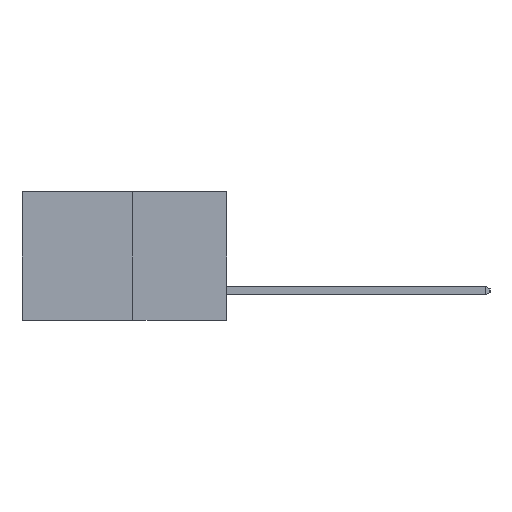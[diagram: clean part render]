
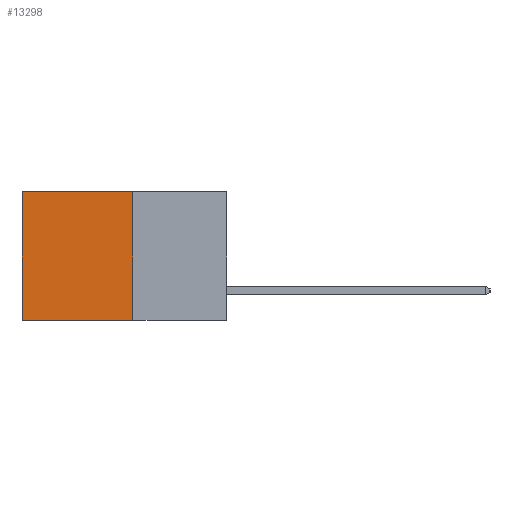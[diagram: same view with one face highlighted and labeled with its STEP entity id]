
A CAD part, left-side view. The second image highlights one B-rep face of the part: STEP entity #13298.
In plain terms, the highlighted planar face has unit normal (-1, 0, 0).
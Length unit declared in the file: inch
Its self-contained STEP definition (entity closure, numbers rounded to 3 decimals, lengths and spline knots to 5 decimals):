
#1461 = CARTESIAN_POINT ( 'NONE',  ( 0.277, 0.59, -0.37 ) ) ;
#2033 = PLANE ( 'NONE',  #18518 ) ;
#2527 = VECTOR ( 'NONE', #5823, 39.37008 ) ;
#3108 = VECTOR ( 'NONE', #15783, 39.37008 ) ;
#3828 = EDGE_CURVE ( 'NONE', #12309, #5552, #7355, .T. ) ;
#5552 = VERTEX_POINT ( 'NONE', #1461 ) ;
#5823 = DIRECTION ( 'NONE',  ( 0., 1., 0. ) ) ;
#6283 = VECTOR ( 'NONE', #8739, 39.37008 ) ;
#6757 = CARTESIAN_POINT ( 'NONE',  ( 0.277, 0.27, -0.37 ) ) ;
#6827 = DIRECTION ( 'NONE',  ( 1., 0., 0. ) ) ;
#7225 = CARTESIAN_POINT ( 'NONE',  ( 0.277, 0.59, -0.37 ) ) ;
#7355 = LINE ( 'NONE', #16213, #3108 ) ;
#7512 = ORIENTED_EDGE ( 'NONE', *, *, #17460, .T. ) ;
#7984 = EDGE_CURVE ( 'NONE', #14740, #12309, #10577, .T. ) ;
#8739 = DIRECTION ( 'NONE',  ( 0., 0., -1. ) ) ;
#8843 = EDGE_LOOP ( 'NONE', ( #11939, #19118, #14989, #7512 ) ) ;
#9005 = CARTESIAN_POINT ( 'NONE',  ( 0.277, 0.27, -0.37 ) ) ;
#10577 = LINE ( 'NONE', #9005, #6283 ) ;
#10618 = LINE ( 'NONE', #7225, #14699 ) ;
#11939 = ORIENTED_EDGE ( 'NONE', *, *, #14161, .T. ) ;
#12121 = DIRECTION ( 'NONE',  ( 0., 0., -1. ) ) ;
#12309 = VERTEX_POINT ( 'NONE', #13579 ) ;
#13160 = CARTESIAN_POINT ( 'NONE',  ( 0.277, 0.59, 0. ) ) ;
#13298 = ADVANCED_FACE ( 'NONE', ( #15226 ), #2033, .F. ) ;
#13319 = VERTEX_POINT ( 'NONE', #13160 ) ;
#13579 = CARTESIAN_POINT ( 'NONE',  ( 0.277, 0.27, -0.37 ) ) ;
#14161 = EDGE_CURVE ( 'NONE', #13319, #5552, #10618, .T. ) ;
#14699 = VECTOR ( 'NONE', #12121, 39.37008 ) ;
#14740 = VERTEX_POINT ( 'NONE', #17809 ) ;
#14989 = ORIENTED_EDGE ( 'NONE', *, *, #7984, .F. ) ;
#15226 = FACE_OUTER_BOUND ( 'NONE', #8843, .T. ) ;
#15783 = DIRECTION ( 'NONE',  ( 0., 1., 0. ) ) ;
#16213 = CARTESIAN_POINT ( 'NONE',  ( 0.277, 0.27, -0.37 ) ) ;
#17460 = EDGE_CURVE ( 'NONE', #14740, #13319, #19628, .T. ) ;
#17716 = DIRECTION ( 'NONE',  ( 0., 0., -1. ) ) ;
#17809 = CARTESIAN_POINT ( 'NONE',  ( 0.277, 0.27, 0. ) ) ;
#18518 = AXIS2_PLACEMENT_3D ( 'NONE', #6757, #6827, #17716 ) ;
#19118 = ORIENTED_EDGE ( 'NONE', *, *, #3828, .F. ) ;
#19628 = LINE ( 'NONE', #19770, #2527 ) ;
#19770 = CARTESIAN_POINT ( 'NONE',  ( 0.277, 0.27, 0. ) ) ;
